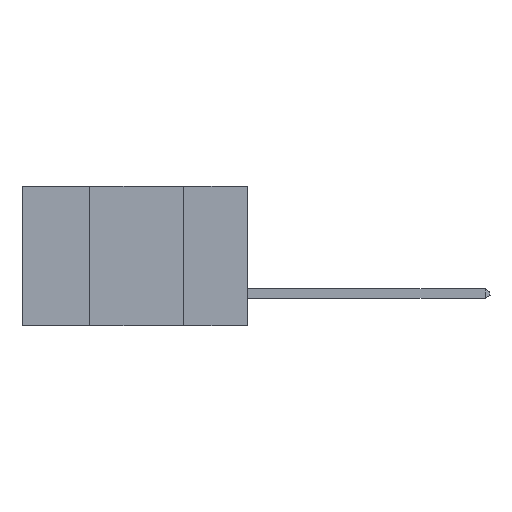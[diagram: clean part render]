
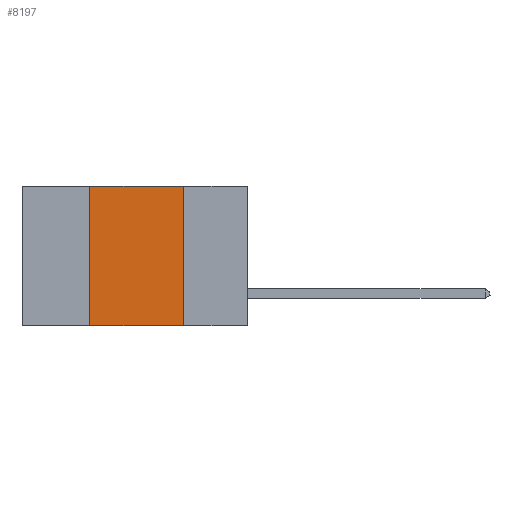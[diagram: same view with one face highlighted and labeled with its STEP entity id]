
A CAD part, left-side view. The second image highlights one B-rep face of the part: STEP entity #8197.
In plain terms, the highlighted planar face has unit normal (-1, 0, 0).
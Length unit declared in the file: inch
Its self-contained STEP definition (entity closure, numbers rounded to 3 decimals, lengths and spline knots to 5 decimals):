
#32 = CARTESIAN_POINT ( 'NONE',  ( 0., 0.42, 0. ) ) ;
#34 = CARTESIAN_POINT ( 'NONE',  ( 0., 0.17, 0. ) ) ;
#429 = ORIENTED_EDGE ( 'NONE', *, *, #3889, .F. ) ;
#957 = DIRECTION ( 'NONE',  ( 0., 0., -1. ) ) ;
#1319 = DIRECTION ( 'NONE',  ( 0., 0., 1. ) ) ;
#1561 = ORIENTED_EDGE ( 'NONE', *, *, #4535, .F. ) ;
#2072 = DIRECTION ( 'NONE',  ( 0., 0., -1. ) ) ;
#2234 = AXIS2_PLACEMENT_3D ( 'NONE', #6200, #6087, #957 ) ;
#2437 = LINE ( 'NONE', #9779, #2568 ) ;
#2568 = VECTOR ( 'NONE', #2072, 39.37008 ) ;
#2603 = VERTEX_POINT ( 'NONE', #32 ) ;
#3101 = EDGE_CURVE ( 'NONE', #5157, #2603, #9584, .T. ) ;
#3258 = FACE_OUTER_BOUND ( 'NONE', #5570, .T. ) ;
#3471 = ORIENTED_EDGE ( 'NONE', *, *, #3101, .F. ) ;
#3886 = VECTOR ( 'NONE', #4782, 39.37008 ) ;
#3889 = EDGE_CURVE ( 'NONE', #9882, #4099, #2437, .T. ) ;
#4099 = VERTEX_POINT ( 'NONE', #9204 ) ;
#4362 = PLANE ( 'NONE',  #2234 ) ;
#4535 = EDGE_CURVE ( 'NONE', #2603, #9882, #5109, .T. ) ;
#4574 = EDGE_CURVE ( 'NONE', #5157, #4099, #9021, .T. ) ;
#4742 = CARTESIAN_POINT ( 'NONE',  ( 0., 0.6, 0. ) ) ;
#4782 = DIRECTION ( 'NONE',  ( 0., -1., 0. ) ) ;
#5109 = LINE ( 'NONE', #4742, #3886 ) ;
#5157 = VERTEX_POINT ( 'NONE', #9336 ) ;
#5570 = EDGE_LOOP ( 'NONE', ( #429, #1561, #3471, #6464 ) ) ;
#5661 = VECTOR ( 'NONE', #1319, 39.37008 ) ;
#6087 = DIRECTION ( 'NONE',  ( 1., 0., 0. ) ) ;
#6200 = CARTESIAN_POINT ( 'NONE',  ( 0., 0.6, 0. ) ) ;
#6464 = ORIENTED_EDGE ( 'NONE', *, *, #4574, .T. ) ;
#7259 = DIRECTION ( 'NONE',  ( 0., -1., 0. ) ) ;
#8110 = CARTESIAN_POINT ( 'NONE',  ( 0., 0.6, -0.37 ) ) ;
#8197 = ADVANCED_FACE ( 'NONE', ( #3258 ), #4362, .F. ) ;
#8964 = CARTESIAN_POINT ( 'NONE',  ( 0., 0.42, 0. ) ) ;
#9021 = LINE ( 'NONE', #8110, #11001 ) ;
#9204 = CARTESIAN_POINT ( 'NONE',  ( 0., 0.17, -0.37 ) ) ;
#9336 = CARTESIAN_POINT ( 'NONE',  ( 0., 0.42, -0.37 ) ) ;
#9584 = LINE ( 'NONE', #8964, #5661 ) ;
#9779 = CARTESIAN_POINT ( 'NONE',  ( 0., 0.17, 0. ) ) ;
#9882 = VERTEX_POINT ( 'NONE', #34 ) ;
#11001 = VECTOR ( 'NONE', #7259, 39.37008 ) ;
